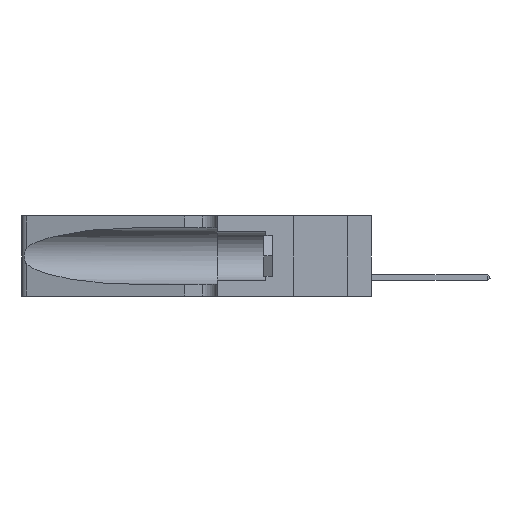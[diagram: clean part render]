
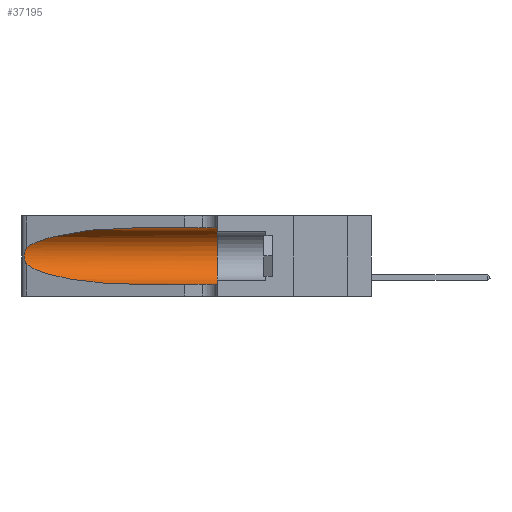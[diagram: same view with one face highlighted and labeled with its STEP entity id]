
A CAD part, left-side view. The second image highlights one B-rep face of the part: STEP entity #37195.
In plain terms, the highlighted cylindrical face has radius 3.308 mm (diameter 6.617 mm), a partial arc.
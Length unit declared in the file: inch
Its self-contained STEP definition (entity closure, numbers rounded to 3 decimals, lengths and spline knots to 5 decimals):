
#81 = VECTOR ( 'NONE', #42993, 39.37008 ) ;
#703 = CARTESIAN_POINT ( 'NONE',  ( 0.1305, 0.35, 0.05475 ) ) ;
#1427 = ORIENTED_EDGE ( 'NONE', *, *, #18666, .T. ) ;
#1892 = CARTESIAN_POINT ( 'NONE',  ( 0.26075, 1.23896, 0.19203 ) ) ;
#2087 = CARTESIAN_POINT ( 'NONE',  ( 0.1305, 1.61858, 0.05475 ) ) ;
#3084 = CARTESIAN_POINT ( 'NONE',  ( 0.25487, 1.22718, 0.22369 ) ) ;
#5248 = CARTESIAN_POINT ( 'NONE',  ( 0.25639, 1.23184, 0.21858 ) ) ;
#5403 = CARTESIAN_POINT ( 'NONE',  ( 0.26075, 1.23896, 0.178 ) ) ;
#5681 = VERTEX_POINT ( 'NONE', #3084 ) ;
#6315 = CARTESIAN_POINT ( 'NONE',  ( 0.25487, 1.22718, 0.14631 ) ) ;
#6372 = EDGE_LOOP ( 'NONE', ( #32145, #28132, #24401, #1427, #14490, #39040 ) ) ;
#6415 = EDGE_CURVE ( 'NONE', #5681, #21515, #12324, .T. ) ;
#8055 = EDGE_CURVE ( 'NONE', #41012, #5681, #29910, .T. ) ;
#9646 = VERTEX_POINT ( 'NONE', #39797 ) ;
#9878 = CARTESIAN_POINT ( 'NONE',  ( 0.2373, 1.15595, 0.28018 ) ) ;
#12280 = CARTESIAN_POINT ( 'NONE',  ( 0.1305, 0.72297, 0.31525 ) ) ;
#12324 = B_SPLINE_CURVE_WITH_KNOTS ( 'NONE', 3,
 ( #30051, #25925, #5248, #36583, #40042, #43522, #1892, #5403, #12391, #23948, #24244, #34758, #13752, #37037 ),
 .UNSPECIFIED., .F., .F.,
 ( 4, 2, 2, 2, 2, 2, 4 ),
 ( 0., 0.00027, 0.00053, 0.00107, 0.0016, 0.00187, 0.00214 ),
 .UNSPECIFIED. ) ;
#12391 = CARTESIAN_POINT ( 'NONE',  ( 0.26017, 1.23833, 0.17102 ) ) ;
#12633 = CARTESIAN_POINT ( 'NONE',  ( 0.2373, 1.15595, 0.08982 ) ) ;
#13752 = CARTESIAN_POINT ( 'NONE',  ( 0.25555, 1.22993, 0.14849 ) ) ;
#14270 = DIRECTION ( 'NONE',  ( 0., 0., 1. ) ) ;
#14490 = ORIENTED_EDGE ( 'NONE', *, *, #17614, .F. ) ;
#14710 =( BOUNDED_CURVE ( )  B_SPLINE_CURVE ( 3, ( #33507, #12633, #18017, #32516 ),
 .UNSPECIFIED., .F., .F. ) 
 B_SPLINE_CURVE_WITH_KNOTS ( ( 4, 4 ),
 ( 3.44316, 4.71239 ),
 .UNSPECIFIED. ) 
 CURVE ( )  GEOMETRIC_REPRESENTATION_ITEM ( )  RATIONAL_B_SPLINE_CURVE ( ( 1., 0.87, 0.87, 1. ) ) 
 REPRESENTATION_ITEM ( '' )  );
#15317 = DIRECTION ( 'NONE',  ( 0., 0., -1. ) ) ;
#16009 = CIRCLE ( 'NONE', #29174, 0.13025 ) ;
#16972 = CARTESIAN_POINT ( 'NONE',  ( 0.18966, 0.96281, 0.31525 ) ) ;
#17336 = DIRECTION ( 'NONE',  ( 0., 1., 0. ) ) ;
#17614 = EDGE_CURVE ( 'NONE', #23272, #44309, #16009, .T. ) ;
#18017 = CARTESIAN_POINT ( 'NONE',  ( 0.18966, 0.96281, 0.05475 ) ) ;
#18368 = CARTESIAN_POINT ( 'NONE',  ( 0.1305, 1.61858, 0.31525 ) ) ;
#18666 = EDGE_CURVE ( 'NONE', #9646, #44309, #37129, .T. ) ;
#19143 = VECTOR ( 'NONE', #33439, 39.37008 ) ;
#20607 = AXIS2_PLACEMENT_3D ( 'NONE', #35887, #25694, #15317 ) ;
#21515 = VERTEX_POINT ( 'NONE', #6315 ) ;
#23272 = VERTEX_POINT ( 'NONE', #36640 ) ;
#23948 = CARTESIAN_POINT ( 'NONE',  ( 0.25856, 1.23593, 0.16098 ) ) ;
#24244 = CARTESIAN_POINT ( 'NONE',  ( 0.25789, 1.23486, 0.15765 ) ) ;
#24401 = ORIENTED_EDGE ( 'NONE', *, *, #24749, .T. ) ;
#24487 = CARTESIAN_POINT ( 'NONE',  ( 0.1305, 0.35, 0.185 ) ) ;
#24749 = EDGE_CURVE ( 'NONE', #21515, #9646, #14710, .T. ) ;
#25694 = DIRECTION ( 'NONE',  ( 0., -1., 0. ) ) ;
#25925 = CARTESIAN_POINT ( 'NONE',  ( 0.25555, 1.22994, 0.2215 ) ) ;
#28132 = ORIENTED_EDGE ( 'NONE', *, *, #6415, .T. ) ;
#29174 = AXIS2_PLACEMENT_3D ( 'NONE', #24487, #17336, #14270 ) ;
#29910 =( BOUNDED_CURVE ( )  B_SPLINE_CURVE ( 3, ( #40863, #16972, #9878, #41296 ),
 .UNSPECIFIED., .F., .F. ) 
 B_SPLINE_CURVE_WITH_KNOTS ( ( 4, 4 ),
 ( 1.5708, 2.84003 ),
 .UNSPECIFIED. ) 
 CURVE ( )  GEOMETRIC_REPRESENTATION_ITEM ( )  RATIONAL_B_SPLINE_CURVE ( ( 1., 0.87, 0.87, 1. ) ) 
 REPRESENTATION_ITEM ( '' )  );
#30051 = CARTESIAN_POINT ( 'NONE',  ( 0.25487, 1.22718, 0.22369 ) ) ;
#32145 = ORIENTED_EDGE ( 'NONE', *, *, #8055, .T. ) ;
#32516 = CARTESIAN_POINT ( 'NONE',  ( 0.1305, 0.72297, 0.05475 ) ) ;
#33439 = DIRECTION ( 'NONE',  ( 0., -1., 0. ) ) ;
#33507 = CARTESIAN_POINT ( 'NONE',  ( 0.25487, 1.22718, 0.14631 ) ) ;
#34758 = CARTESIAN_POINT ( 'NONE',  ( 0.25639, 1.23186, 0.15144 ) ) ;
#35887 = CARTESIAN_POINT ( 'NONE',  ( 0.1305, 1.61858, 0.185 ) ) ;
#36583 = CARTESIAN_POINT ( 'NONE',  ( 0.25787, 1.23484, 0.2124 ) ) ;
#36640 = CARTESIAN_POINT ( 'NONE',  ( 0.1305, 0.35, 0.31525 ) ) ;
#37037 = CARTESIAN_POINT ( 'NONE',  ( 0.25487, 1.22718, 0.14631 ) ) ;
#37114 = LINE ( 'NONE', #18368, #81 ) ;
#37129 = LINE ( 'NONE', #2087, #19143 ) ;
#37195 = ADVANCED_FACE ( 'NONE', ( #40815 ), #44065, .F. ) ;
#39040 = ORIENTED_EDGE ( 'NONE', *, *, #42144, .F. ) ;
#39797 = CARTESIAN_POINT ( 'NONE',  ( 0.1305, 0.72297, 0.05475 ) ) ;
#40042 = CARTESIAN_POINT ( 'NONE',  ( 0.25854, 1.2359, 0.20912 ) ) ;
#40815 = FACE_OUTER_BOUND ( 'NONE', #6372, .T. ) ;
#40863 = CARTESIAN_POINT ( 'NONE',  ( 0.1305, 0.72297, 0.31525 ) ) ;
#41012 = VERTEX_POINT ( 'NONE', #12280 ) ;
#41296 = CARTESIAN_POINT ( 'NONE',  ( 0.25487, 1.22718, 0.22369 ) ) ;
#42144 = EDGE_CURVE ( 'NONE', #41012, #23272, #37114, .T. ) ;
#42993 = DIRECTION ( 'NONE',  ( 0., -1., 0. ) ) ;
#43522 = CARTESIAN_POINT ( 'NONE',  ( 0.26018, 1.23835, 0.19895 ) ) ;
#44065 = CYLINDRICAL_SURFACE ( 'NONE', #20607, 0.13025 ) ;
#44309 = VERTEX_POINT ( 'NONE', #703 ) ;
